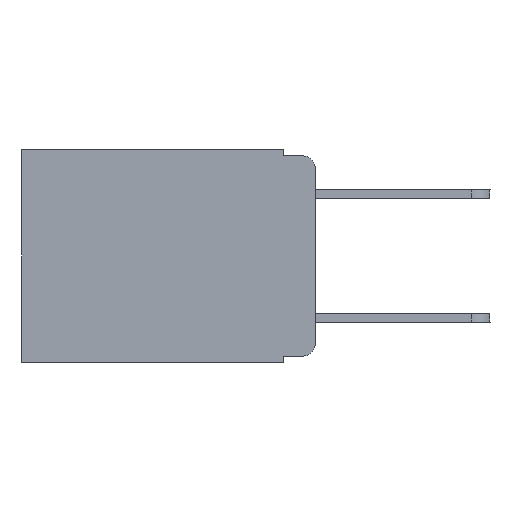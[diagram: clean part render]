
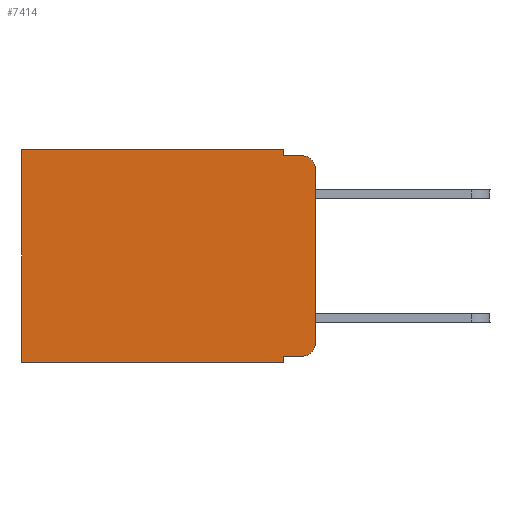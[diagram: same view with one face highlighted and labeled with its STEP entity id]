
A CAD part, left-side view. The second image highlights one B-rep face of the part: STEP entity #7414.
In plain terms, the highlighted planar face has unit normal (-1, 0, 0).
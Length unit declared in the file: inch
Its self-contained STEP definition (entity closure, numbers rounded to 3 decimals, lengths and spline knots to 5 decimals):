
#646 = VECTOR ( 'NONE', #15476, 39.37008 ) ;
#2007 = ORIENTED_EDGE ( 'NONE', *, *, #7331, .F. ) ;
#2027 = LINE ( 'NONE', #5563, #19929 ) ;
#2112 = DIRECTION ( 'NONE',  ( -1., 0., 0. ) ) ;
#2179 = ORIENTED_EDGE ( 'NONE', *, *, #12374, .F. ) ;
#2551 = CARTESIAN_POINT ( 'NONE',  ( 0.298, 0.473, -0.343 ) ) ;
#2722 = VECTOR ( 'NONE', #19698, 39.37008 ) ;
#2803 = ORIENTED_EDGE ( 'NONE', *, *, #12757, .T. ) ;
#2873 = DIRECTION ( 'NONE',  ( 0., 0., -1. ) ) ;
#3038 = VERTEX_POINT ( 'NONE', #19107 ) ;
#3502 = CARTESIAN_POINT ( 'NONE',  ( 0.298, 0.051, 0. ) ) ;
#3846 = VECTOR ( 'NONE', #6027, 39.37008 ) ;
#3847 = ORIENTED_EDGE ( 'NONE', *, *, #4495, .T. ) ;
#4495 = EDGE_CURVE ( 'NONE', #12175, #13919, #21539, .T. ) ;
#4979 = VECTOR ( 'NONE', #2873, 39.37008 ) ;
#5093 = DIRECTION ( 'NONE',  ( -1., 0., 0. ) ) ;
#5111 = ORIENTED_EDGE ( 'NONE', *, *, #12972, .F. ) ;
#5125 = VECTOR ( 'NONE', #21096, 39.37008 ) ;
#5202 = EDGE_CURVE ( 'NONE', #13919, #6505, #18132, .T. ) ;
#5388 = VERTEX_POINT ( 'NONE', #20399 ) ;
#5563 = CARTESIAN_POINT ( 'NONE',  ( 0.298, 0.051, -0.01 ) ) ;
#5585 = CARTESIAN_POINT ( 'NONE',  ( 0.298, 0.051, -0.01 ) ) ;
#6027 = DIRECTION ( 'NONE',  ( 0., 0., -1. ) ) ;
#6116 = CIRCLE ( 'NONE', #18796, 0.02 ) ;
#6451 = ORIENTED_EDGE ( 'NONE', *, *, #7339, .F. ) ;
#6505 = VERTEX_POINT ( 'NONE', #2551 ) ;
#6705 = ORIENTED_EDGE ( 'NONE', *, *, #16843, .F. ) ;
#7002 = EDGE_CURVE ( 'NONE', #9381, #21584, #20906, .T. ) ;
#7233 = DIRECTION ( 'NONE',  ( 0., 0., -1. ) ) ;
#7331 = EDGE_CURVE ( 'NONE', #9381, #16706, #20127, .T. ) ;
#7339 = EDGE_CURVE ( 'NONE', #5388, #19868, #16240, .T. ) ;
#7414 = ADVANCED_FACE ( 'NONE', ( #14889 ), #19779, .F. ) ;
#7554 = CARTESIAN_POINT ( 'NONE',  ( 0.298, 0.02, -0.01 ) ) ;
#7941 = CARTESIAN_POINT ( 'NONE',  ( 0.298, 0., 0. ) ) ;
#8168 = AXIS2_PLACEMENT_3D ( 'NONE', #13305, #5093, #18979 ) ;
#8531 = LINE ( 'NONE', #17180, #646 ) ;
#8780 = LINE ( 'NONE', #18804, #5125 ) ;
#9278 = AXIS2_PLACEMENT_3D ( 'NONE', #18196, #16123, #21395 ) ;
#9381 = VERTEX_POINT ( 'NONE', #21405 ) ;
#9582 = CARTESIAN_POINT ( 'NONE',  ( 0.298, 0.473, 0. ) ) ;
#10414 = VECTOR ( 'NONE', #15897, 39.37008 ) ;
#10883 = LINE ( 'NONE', #21158, #10414 ) ;
#12090 = CARTESIAN_POINT ( 'NONE',  ( 0.298, 0.02, -0.313 ) ) ;
#12175 = VERTEX_POINT ( 'NONE', #3502 ) ;
#12256 = DIRECTION ( 'NONE',  ( 0., -1., 0. ) ) ;
#12374 = EDGE_CURVE ( 'NONE', #19868, #6505, #10883, .T. ) ;
#12757 = EDGE_CURVE ( 'NONE', #3038, #16706, #6116, .T. ) ;
#12972 = EDGE_CURVE ( 'NONE', #17950, #21584, #2027, .T. ) ;
#13305 = CARTESIAN_POINT ( 'NONE',  ( 0.298, 0.02, -0.03 ) ) ;
#13919 = VERTEX_POINT ( 'NONE', #22244 ) ;
#14534 = ORIENTED_EDGE ( 'NONE', *, *, #7002, .T. ) ;
#14771 = ORIENTED_EDGE ( 'NONE', *, *, #20935, .T. ) ;
#14889 = FACE_OUTER_BOUND ( 'NONE', #21688, .T. ) ;
#15476 = DIRECTION ( 'NONE',  ( 0., -1., 0. ) ) ;
#15897 = DIRECTION ( 'NONE',  ( 0., 1., 0. ) ) ;
#16123 = DIRECTION ( 'NONE',  ( 1., 0., 0. ) ) ;
#16240 = LINE ( 'NONE', #21734, #3846 ) ;
#16706 = VERTEX_POINT ( 'NONE', #22231 ) ;
#16843 = EDGE_CURVE ( 'NONE', #12175, #17950, #8780, .T. ) ;
#17180 = CARTESIAN_POINT ( 'NONE',  ( 0.298, 0.051, -0.333 ) ) ;
#17950 = VERTEX_POINT ( 'NONE', #5585 ) ;
#18132 = LINE ( 'NONE', #9582, #4979 ) ;
#18196 = CARTESIAN_POINT ( 'NONE',  ( 0.298, 0., 0. ) ) ;
#18746 = ORIENTED_EDGE ( 'NONE', *, *, #5202, .T. ) ;
#18796 = AXIS2_PLACEMENT_3D ( 'NONE', #12090, #2112, #7233 ) ;
#18804 = CARTESIAN_POINT ( 'NONE',  ( 0.298, 0.051, 0. ) ) ;
#18979 = DIRECTION ( 'NONE',  ( 0., 0., -1. ) ) ;
#19087 = VECTOR ( 'NONE', #19668, 39.37008 ) ;
#19107 = CARTESIAN_POINT ( 'NONE',  ( 0.298, 0.02, -0.333 ) ) ;
#19668 = DIRECTION ( 'NONE',  ( 0., 0., -1. ) ) ;
#19698 = DIRECTION ( 'NONE',  ( 0., 1., 0. ) ) ;
#19779 = PLANE ( 'NONE',  #9278 ) ;
#19868 = VERTEX_POINT ( 'NONE', #21398 ) ;
#19929 = VECTOR ( 'NONE', #12256, 39.37008 ) ;
#20127 = LINE ( 'NONE', #7941, #19087 ) ;
#20399 = CARTESIAN_POINT ( 'NONE',  ( 0.298, 0.051, -0.333 ) ) ;
#20906 = CIRCLE ( 'NONE', #8168, 0.02 ) ;
#20935 = EDGE_CURVE ( 'NONE', #5388, #3038, #8531, .T. ) ;
#21096 = DIRECTION ( 'NONE',  ( 0., 0., -1. ) ) ;
#21158 = CARTESIAN_POINT ( 'NONE',  ( 0.298, 0., -0.343 ) ) ;
#21395 = DIRECTION ( 'NONE',  ( 0., 0., -1. ) ) ;
#21398 = CARTESIAN_POINT ( 'NONE',  ( 0.298, 0.051, -0.343 ) ) ;
#21405 = CARTESIAN_POINT ( 'NONE',  ( 0.298, 0., -0.03 ) ) ;
#21539 = LINE ( 'NONE', #21650, #2722 ) ;
#21584 = VERTEX_POINT ( 'NONE', #7554 ) ;
#21650 = CARTESIAN_POINT ( 'NONE',  ( 0.298, 0., 0. ) ) ;
#21688 = EDGE_LOOP ( 'NONE', ( #2007, #14534, #5111, #6705, #3847, #18746, #2179, #6451, #14771, #2803 ) ) ;
#21734 = CARTESIAN_POINT ( 'NONE',  ( 0.298, 0.051, 0. ) ) ;
#22231 = CARTESIAN_POINT ( 'NONE',  ( 0.298, 0., -0.313 ) ) ;
#22244 = CARTESIAN_POINT ( 'NONE',  ( 0.298, 0.473, 0. ) ) ;
